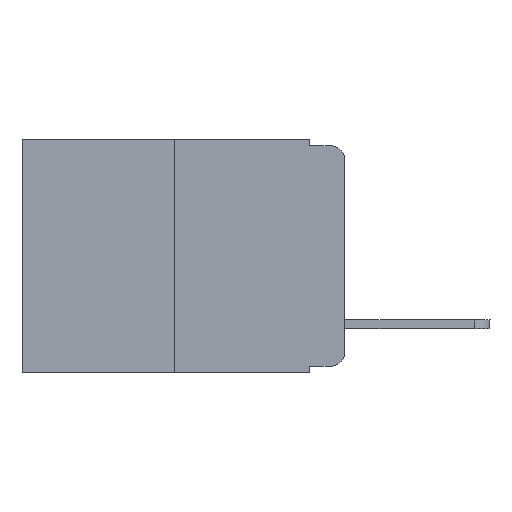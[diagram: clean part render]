
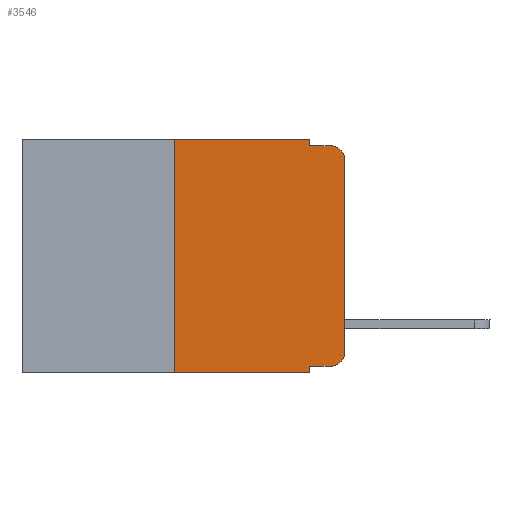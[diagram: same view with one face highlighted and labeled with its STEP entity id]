
A CAD part, left-side view. The second image highlights one B-rep face of the part: STEP entity #3546.
In plain terms, the highlighted planar face has unit normal (-1, 0, 0).
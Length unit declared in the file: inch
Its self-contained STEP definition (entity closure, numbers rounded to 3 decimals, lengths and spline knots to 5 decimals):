
#59 = DIRECTION ( 'NONE',  ( 0., -1., 0. ) ) ;
#176 = DIRECTION ( 'NONE',  ( 0., 0., -1. ) ) ;
#391 = CIRCLE ( 'NONE', #6800, 0.02 ) ;
#395 = LINE ( 'NONE', #3743, #9227 ) ;
#499 = CARTESIAN_POINT ( 'NONE',  ( 0., 0.25, 0. ) ) ;
#530 = VECTOR ( 'NONE', #4017, 39.37008 ) ;
#591 = LINE ( 'NONE', #696, #530 ) ;
#696 = CARTESIAN_POINT ( 'NONE',  ( 0., 0.051, -0.01 ) ) ;
#828 = EDGE_CURVE ( 'NONE', #4845, #8025, #2310, .T. ) ;
#864 = VERTEX_POINT ( 'NONE', #4268 ) ;
#937 = PLANE ( 'NONE',  #8853 ) ;
#997 = VECTOR ( 'NONE', #3001, 39.37008 ) ;
#1037 = ORIENTED_EDGE ( 'NONE', *, *, #7991, .F. ) ;
#1100 = DIRECTION ( 'NONE',  ( 0., -1., 0. ) ) ;
#1152 = CARTESIAN_POINT ( 'NONE',  ( 0., 0.051, 0. ) ) ;
#1296 = CARTESIAN_POINT ( 'NONE',  ( 0., 0.051, 0. ) ) ;
#1450 = EDGE_CURVE ( 'NONE', #4869, #8025, #3232, .T. ) ;
#1774 = FACE_OUTER_BOUND ( 'NONE', #10799, .T. ) ;
#1934 = EDGE_CURVE ( 'NONE', #2636, #864, #391, .T. ) ;
#2036 = EDGE_CURVE ( 'NONE', #4869, #7560, #6182, .T. ) ;
#2310 = LINE ( 'NONE', #6821, #6978 ) ;
#2354 = DIRECTION ( 'NONE',  ( -1., 0., 0. ) ) ;
#2497 = CARTESIAN_POINT ( 'NONE',  ( 0., 0.051, 0. ) ) ;
#2557 = AXIS2_PLACEMENT_3D ( 'NONE', #7299, #2354, #8083 ) ;
#2636 = VERTEX_POINT ( 'NONE', #3938 ) ;
#3001 = DIRECTION ( 'NONE',  ( 0., 0., -1. ) ) ;
#3164 = VERTEX_POINT ( 'NONE', #7768 ) ;
#3232 = LINE ( 'NONE', #2497, #5403 ) ;
#3283 = ORIENTED_EDGE ( 'NONE', *, *, #7238, .T. ) ;
#3546 = ADVANCED_FACE ( 'NONE', ( #1774 ), #937, .F. ) ;
#3743 = CARTESIAN_POINT ( 'NONE',  ( 0., 0.473, 0. ) ) ;
#3892 = ORIENTED_EDGE ( 'NONE', *, *, #8163, .F. ) ;
#3938 = CARTESIAN_POINT ( 'NONE',  ( 0., 0., -0.03 ) ) ;
#4017 = DIRECTION ( 'NONE',  ( 0., -1., 0. ) ) ;
#4062 = LINE ( 'NONE', #1296, #997 ) ;
#4120 = ORIENTED_EDGE ( 'NONE', *, *, #6317, .T. ) ;
#4247 = EDGE_CURVE ( 'NONE', #7576, #3164, #4062, .T. ) ;
#4268 = CARTESIAN_POINT ( 'NONE',  ( 0., 0.02, -0.01 ) ) ;
#4302 = CARTESIAN_POINT ( 'NONE',  ( 0., 0.473, 0. ) ) ;
#4560 = LINE ( 'NONE', #7279, #10334 ) ;
#4845 = VERTEX_POINT ( 'NONE', #5068 ) ;
#4857 = ORIENTED_EDGE ( 'NONE', *, *, #10502, .F. ) ;
#4869 = VERTEX_POINT ( 'NONE', #6132 ) ;
#4890 = CARTESIAN_POINT ( 'NONE',  ( 0., 0., -0.313 ) ) ;
#5032 = DIRECTION ( 'NONE',  ( 0., -1., 0. ) ) ;
#5068 = CARTESIAN_POINT ( 'NONE',  ( 0., 0.25, -0.343 ) ) ;
#5403 = VECTOR ( 'NONE', #7507, 39.37008 ) ;
#5500 = VERTEX_POINT ( 'NONE', #4890 ) ;
#5582 = LINE ( 'NONE', #9890, #7016 ) ;
#6132 = CARTESIAN_POINT ( 'NONE',  ( 0., 0.051, -0.333 ) ) ;
#6182 = LINE ( 'NONE', #8568, #8523 ) ;
#6205 = ORIENTED_EDGE ( 'NONE', *, *, #4247, .F. ) ;
#6317 = EDGE_CURVE ( 'NONE', #7560, #5500, #7351, .T. ) ;
#6416 = VERTEX_POINT ( 'NONE', #499 ) ;
#6502 = ORIENTED_EDGE ( 'NONE', *, *, #1934, .T. ) ;
#6599 = DIRECTION ( 'NONE',  ( 0., 0., 1. ) ) ;
#6800 = AXIS2_PLACEMENT_3D ( 'NONE', #9594, #10260, #176 ) ;
#6801 = DIRECTION ( 'NONE',  ( 1., 0., 0. ) ) ;
#6821 = CARTESIAN_POINT ( 'NONE',  ( 0., 0.473, -0.343 ) ) ;
#6978 = VECTOR ( 'NONE', #5032, 39.37008 ) ;
#7016 = VECTOR ( 'NONE', #6599, 39.37008 ) ;
#7238 = EDGE_CURVE ( 'NONE', #5500, #2636, #5582, .T. ) ;
#7279 = CARTESIAN_POINT ( 'NONE',  ( 0., 0.25, 0. ) ) ;
#7299 = CARTESIAN_POINT ( 'NONE',  ( 0., 0.02, -0.313 ) ) ;
#7351 = CIRCLE ( 'NONE', #2557, 0.02 ) ;
#7507 = DIRECTION ( 'NONE',  ( 0., 0., -1. ) ) ;
#7560 = VERTEX_POINT ( 'NONE', #9801 ) ;
#7576 = VERTEX_POINT ( 'NONE', #1152 ) ;
#7768 = CARTESIAN_POINT ( 'NONE',  ( 0., 0.051, -0.01 ) ) ;
#7991 = EDGE_CURVE ( 'NONE', #4845, #6416, #4560, .T. ) ;
#8001 = CARTESIAN_POINT ( 'NONE',  ( 0., 0.051, -0.343 ) ) ;
#8025 = VERTEX_POINT ( 'NONE', #8001 ) ;
#8083 = DIRECTION ( 'NONE',  ( 0., 0., -1. ) ) ;
#8163 = EDGE_CURVE ( 'NONE', #3164, #864, #591, .T. ) ;
#8338 = ORIENTED_EDGE ( 'NONE', *, *, #828, .T. ) ;
#8458 = DIRECTION ( 'NONE',  ( 0., 0., -1. ) ) ;
#8523 = VECTOR ( 'NONE', #59, 39.37008 ) ;
#8568 = CARTESIAN_POINT ( 'NONE',  ( 0., 0.051, -0.333 ) ) ;
#8853 = AXIS2_PLACEMENT_3D ( 'NONE', #4302, #6801, #8458 ) ;
#9227 = VECTOR ( 'NONE', #1100, 39.37008 ) ;
#9457 = ORIENTED_EDGE ( 'NONE', *, *, #1450, .F. ) ;
#9594 = CARTESIAN_POINT ( 'NONE',  ( 0., 0.02, -0.03 ) ) ;
#9801 = CARTESIAN_POINT ( 'NONE',  ( 0., 0.02, -0.333 ) ) ;
#9890 = CARTESIAN_POINT ( 'NONE',  ( 0., 0., 0. ) ) ;
#10050 = ORIENTED_EDGE ( 'NONE', *, *, #2036, .T. ) ;
#10260 = DIRECTION ( 'NONE',  ( -1., 0., 0. ) ) ;
#10334 = VECTOR ( 'NONE', #10515, 39.37008 ) ;
#10502 = EDGE_CURVE ( 'NONE', #6416, #7576, #395, .T. ) ;
#10515 = DIRECTION ( 'NONE',  ( 0., 0., 1. ) ) ;
#10799 = EDGE_LOOP ( 'NONE', ( #3283, #6502, #3892, #6205, #4857, #1037, #8338, #9457, #10050, #4120 ) ) ;
